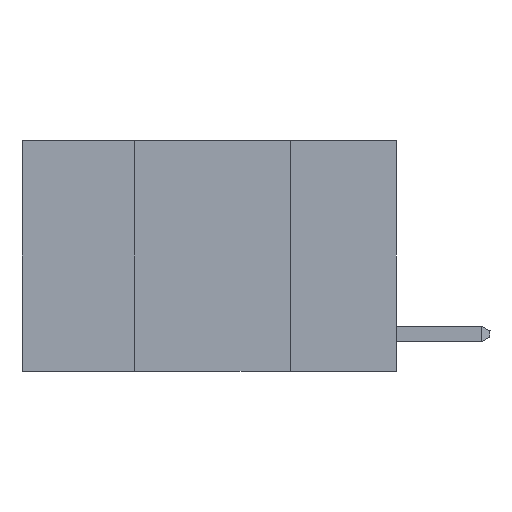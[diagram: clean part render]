
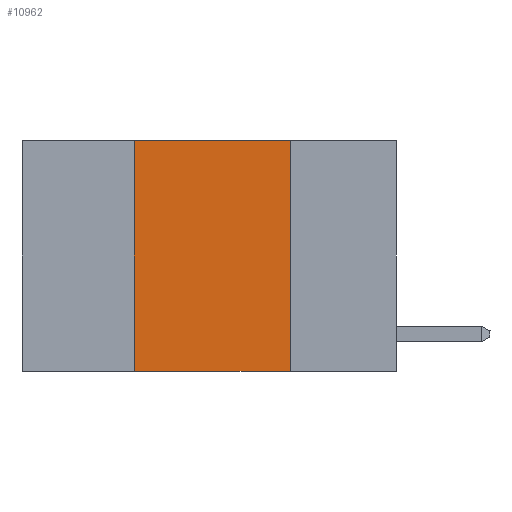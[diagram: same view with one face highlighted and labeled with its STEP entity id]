
A CAD part, left-side view. The second image highlights one B-rep face of the part: STEP entity #10962.
In plain terms, the highlighted planar face has unit normal (-1, 0, 0).
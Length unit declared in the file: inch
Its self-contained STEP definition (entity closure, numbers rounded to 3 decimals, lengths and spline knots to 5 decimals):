
#2452 = DIRECTION ( 'NONE',  ( 0., 0., 1. ) ) ;
#2669 = VECTOR ( 'NONE', #2452, 39.37008 ) ;
#2987 = DIRECTION ( 'NONE',  ( 0., -1., 0. ) ) ;
#3324 = LINE ( 'NONE', #22506, #23754 ) ;
#3613 = LINE ( 'NONE', #14453, #14340 ) ;
#3822 = EDGE_CURVE ( 'NONE', #14497, #16224, #11008, .T. ) ;
#3969 = CARTESIAN_POINT ( 'NONE',  ( 0., 0.17, -0.37 ) ) ;
#4911 = AXIS2_PLACEMENT_3D ( 'NONE', #17263, #6199, #21660 ) ;
#5030 = EDGE_LOOP ( 'NONE', ( #23965, #10094, #28478, #6881 ) ) ;
#6199 = DIRECTION ( 'NONE',  ( 1., 0., 0. ) ) ;
#6881 = ORIENTED_EDGE ( 'NONE', *, *, #11318, .T. ) ;
#7335 = CARTESIAN_POINT ( 'NONE',  ( 0., 0.6, 0. ) ) ;
#10094 = ORIENTED_EDGE ( 'NONE', *, *, #10673, .F. ) ;
#10603 = CARTESIAN_POINT ( 'NONE',  ( 0., 0.17, 0. ) ) ;
#10673 = EDGE_CURVE ( 'NONE', #16224, #13399, #19370, .T. ) ;
#10962 = ADVANCED_FACE ( 'NONE', ( #13780 ), #25982, .F. ) ;
#11008 = LINE ( 'NONE', #20186, #2669 ) ;
#11318 = EDGE_CURVE ( 'NONE', #14497, #20518, #3324, .T. ) ;
#11983 = DIRECTION ( 'NONE',  ( 0., -1., 0. ) ) ;
#12891 = EDGE_CURVE ( 'NONE', #13399, #20518, #3613, .T. ) ;
#13399 = VERTEX_POINT ( 'NONE', #10603 ) ;
#13780 = FACE_OUTER_BOUND ( 'NONE', #5030, .T. ) ;
#14340 = VECTOR ( 'NONE', #23499, 39.37008 ) ;
#14453 = CARTESIAN_POINT ( 'NONE',  ( 0., 0.17, 0. ) ) ;
#14497 = VERTEX_POINT ( 'NONE', #22283 ) ;
#16224 = VERTEX_POINT ( 'NONE', #19041 ) ;
#17263 = CARTESIAN_POINT ( 'NONE',  ( 0., 0.6, 0. ) ) ;
#18293 = VECTOR ( 'NONE', #11983, 39.37008 ) ;
#19041 = CARTESIAN_POINT ( 'NONE',  ( 0., 0.42, 0. ) ) ;
#19370 = LINE ( 'NONE', #7335, #18293 ) ;
#20186 = CARTESIAN_POINT ( 'NONE',  ( 0., 0.42, 0. ) ) ;
#20518 = VERTEX_POINT ( 'NONE', #3969 ) ;
#21660 = DIRECTION ( 'NONE',  ( 0., 0., -1. ) ) ;
#22283 = CARTESIAN_POINT ( 'NONE',  ( 0., 0.42, -0.37 ) ) ;
#22506 = CARTESIAN_POINT ( 'NONE',  ( 0., 0.6, -0.37 ) ) ;
#23499 = DIRECTION ( 'NONE',  ( 0., 0., -1. ) ) ;
#23754 = VECTOR ( 'NONE', #2987, 39.37008 ) ;
#23965 = ORIENTED_EDGE ( 'NONE', *, *, #12891, .F. ) ;
#25982 = PLANE ( 'NONE',  #4911 ) ;
#28478 = ORIENTED_EDGE ( 'NONE', *, *, #3822, .F. ) ;
